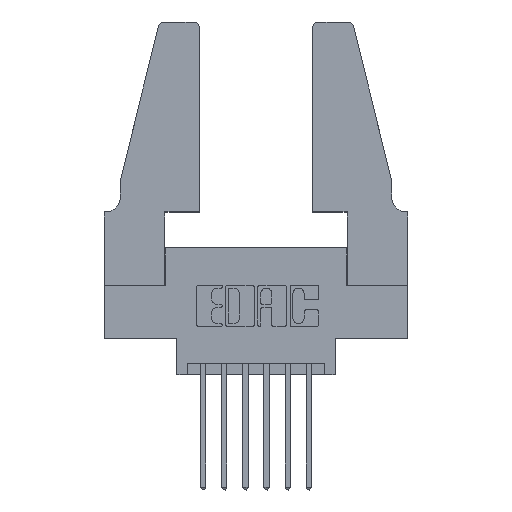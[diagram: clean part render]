
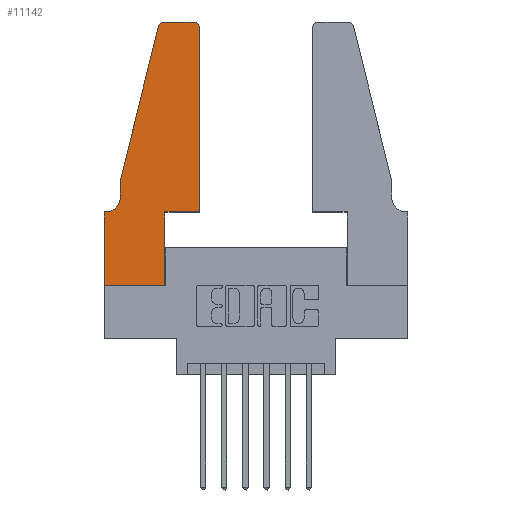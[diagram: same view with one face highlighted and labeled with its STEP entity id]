
A CAD part, top view. The second image highlights one B-rep face of the part: STEP entity #11142.
In plain terms, the highlighted planar face has unit normal (0, 0, 1).
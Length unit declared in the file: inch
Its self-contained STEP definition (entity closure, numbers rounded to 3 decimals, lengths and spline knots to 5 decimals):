
#231 = EDGE_CURVE ( 'NONE', #10431, #8152, #8017, .T. ) ;
#592 = VECTOR ( 'NONE', #11217, 39.37008 ) ;
#640 = DIRECTION ( 'NONE',  ( 0., 0., 1. ) ) ;
#743 = EDGE_CURVE ( 'NONE', #6571, #9268, #5655, .T. ) ;
#839 = CARTESIAN_POINT ( 'NONE',  ( 0.284, 1.22, 0.37 ) ) ;
#926 = EDGE_CURVE ( 'NONE', #6326, #11310, #8406, .T. ) ;
#970 = CARTESIAN_POINT ( 'NONE',  ( 0.0055, 0.42, 0.37 ) ) ;
#1036 = ORIENTED_EDGE ( 'NONE', *, *, #231, .T. ) ;
#1042 = VECTOR ( 'NONE', #9779, 39.37008 ) ;
#1610 = VERTEX_POINT ( 'NONE', #11147 ) ;
#1614 = FACE_OUTER_BOUND ( 'NONE', #6692, .T. ) ;
#1713 = DIRECTION ( 'NONE',  ( 0., 0., 1. ) ) ;
#1777 = DIRECTION ( 'NONE',  ( 1., 0., 0. ) ) ;
#1792 = VERTEX_POINT ( 'NONE', #5857 ) ;
#1813 = VERTEX_POINT ( 'NONE', #5241 ) ;
#1886 = DIRECTION ( 'NONE',  ( -0.239, -0.971, 0. ) ) ;
#1920 = DIRECTION ( 'NONE',  ( -1., 0., 0. ) ) ;
#1927 = CARTESIAN_POINT ( 'NONE',  ( 0.4505, 0.35, 0.37 ) ) ;
#1946 = EDGE_CURVE ( 'NONE', #9268, #1813, #5762, .T. ) ;
#2195 = VERTEX_POINT ( 'NONE', #5952 ) ;
#2462 = VECTOR ( 'NONE', #10970, 39.37008 ) ;
#2817 = EDGE_CURVE ( 'NONE', #7672, #1792, #4414, .T. ) ;
#2962 = ORIENTED_EDGE ( 'NONE', *, *, #7625, .T. ) ;
#3680 = VECTOR ( 'NONE', #4369, 39.37008 ) ;
#3730 = EDGE_CURVE ( 'NONE', #1792, #2195, #11265, .T. ) ;
#3849 = ORIENTED_EDGE ( 'NONE', *, *, #6217, .T. ) ;
#4110 = VECTOR ( 'NONE', #5999, 39.37008 ) ;
#4369 = DIRECTION ( 'NONE',  ( 0., -1., 0. ) ) ;
#4414 = LINE ( 'NONE', #6388, #4110 ) ;
#4507 = EDGE_CURVE ( 'NONE', #1610, #10431, #7741, .T. ) ;
#4512 = CARTESIAN_POINT ( 'NONE',  ( 0.0755, 0.5, 0.37 ) ) ;
#4696 = VERTEX_POINT ( 'NONE', #9492 ) ;
#4746 = ORIENTED_EDGE ( 'NONE', *, *, #2817, .T. ) ;
#5241 = CARTESIAN_POINT ( 'NONE',  ( 0., 0., 0.37 ) ) ;
#5282 = CARTESIAN_POINT ( 'NONE',  ( 0.0755, 0.5, 0.37 ) ) ;
#5295 = CARTESIAN_POINT ( 'NONE',  ( 0., 0.35, 0.37 ) ) ;
#5655 = LINE ( 'NONE', #8463, #592 ) ;
#5685 = AXIS2_PLACEMENT_3D ( 'NONE', #7307, #1713, #8178 ) ;
#5762 = LINE ( 'NONE', #6848, #10183 ) ;
#5857 = CARTESIAN_POINT ( 'NONE',  ( 0.4505, 1.22, 0.37 ) ) ;
#5952 = CARTESIAN_POINT ( 'NONE',  ( 0.4205, 1.25, 0.37 ) ) ;
#5999 = DIRECTION ( 'NONE',  ( 0., 1., 0. ) ) ;
#6182 = LINE ( 'NONE', #5282, #3680 ) ;
#6217 = EDGE_CURVE ( 'NONE', #8152, #4696, #6182, .T. ) ;
#6241 = AXIS2_PLACEMENT_3D ( 'NONE', #839, #7368, #1777 ) ;
#6295 = CARTESIAN_POINT ( 'NONE',  ( 0.4205, 1.22, 0.37 ) ) ;
#6326 = VERTEX_POINT ( 'NONE', #6355 ) ;
#6337 = ORIENTED_EDGE ( 'NONE', *, *, #11269, .T. ) ;
#6355 = CARTESIAN_POINT ( 'NONE',  ( 0.2865, 0., 0.37 ) ) ;
#6388 = CARTESIAN_POINT ( 'NONE',  ( 0.4505, 0.35, 0.37 ) ) ;
#6549 = VECTOR ( 'NONE', #6674, 39.37008 ) ;
#6561 = CARTESIAN_POINT ( 'NONE',  ( 0.2605, 1.25, 0.37 ) ) ;
#6571 = VERTEX_POINT ( 'NONE', #11098 ) ;
#6674 = DIRECTION ( 'NONE',  ( 1., 0., 0. ) ) ;
#6692 = EDGE_LOOP ( 'NONE', ( #2962, #10195, #1036, #3849, #6337, #11044, #8953, #11326, #9220, #11595, #4746, #7190 ) ) ;
#6774 = VECTOR ( 'NONE', #7971, 39.37008 ) ;
#6848 = CARTESIAN_POINT ( 'NONE',  ( 0., 0., 0.37 ) ) ;
#7104 = CARTESIAN_POINT ( 'NONE',  ( 0.4505, 0.35, 0.37 ) ) ;
#7190 = ORIENTED_EDGE ( 'NONE', *, *, #3730, .T. ) ;
#7198 = DIRECTION ( 'NONE',  ( 1., 0., 0. ) ) ;
#7307 = CARTESIAN_POINT ( 'NONE',  ( 0., 0.35, 0.37 ) ) ;
#7368 = DIRECTION ( 'NONE',  ( 0., 0., 1. ) ) ;
#7391 = LINE ( 'NONE', #6561, #2462 ) ;
#7485 = AXIS2_PLACEMENT_3D ( 'NONE', #6295, #640, #7198 ) ;
#7489 = DIRECTION ( 'NONE',  ( 0., 0., -1. ) ) ;
#7569 = CIRCLE ( 'NONE', #11024, 0.07 ) ;
#7625 = EDGE_CURVE ( 'NONE', #2195, #1610, #7391, .T. ) ;
#7672 = VERTEX_POINT ( 'NONE', #1927 ) ;
#7702 = EDGE_CURVE ( 'NONE', #1813, #6326, #9426, .T. ) ;
#7741 = CIRCLE ( 'NONE', #6241, 0.03 ) ;
#7971 = DIRECTION ( 'NONE',  ( 1., 0., 0. ) ) ;
#8017 = LINE ( 'NONE', #4512, #10084 ) ;
#8152 = VERTEX_POINT ( 'NONE', #11727 ) ;
#8178 = DIRECTION ( 'NONE',  ( 1., 0., 0. ) ) ;
#8406 = LINE ( 'NONE', #10836, #1042 ) ;
#8463 = CARTESIAN_POINT ( 'NONE',  ( 0.0755, 0.35, 0.37 ) ) ;
#8953 = ORIENTED_EDGE ( 'NONE', *, *, #1946, .T. ) ;
#9108 = LINE ( 'NONE', #7104, #6774 ) ;
#9220 = ORIENTED_EDGE ( 'NONE', *, *, #926, .T. ) ;
#9268 = VERTEX_POINT ( 'NONE', #5295 ) ;
#9426 = LINE ( 'NONE', #10181, #6549 ) ;
#9492 = CARTESIAN_POINT ( 'NONE',  ( 0.0755, 0.42, 0.37 ) ) ;
#9779 = DIRECTION ( 'NONE',  ( 0., 1., 0. ) ) ;
#9799 = EDGE_CURVE ( 'NONE', #11310, #7672, #9108, .T. ) ;
#10084 = VECTOR ( 'NONE', #1886, 39.37008 ) ;
#10178 = CARTESIAN_POINT ( 'NONE',  ( 0.2865, 0.35, 0.37 ) ) ;
#10181 = CARTESIAN_POINT ( 'NONE',  ( 0., 0., 0.37 ) ) ;
#10183 = VECTOR ( 'NONE', #11556, 39.37008 ) ;
#10195 = ORIENTED_EDGE ( 'NONE', *, *, #4507, .T. ) ;
#10431 = VERTEX_POINT ( 'NONE', #10592 ) ;
#10592 = CARTESIAN_POINT ( 'NONE',  ( 0.25487, 1.22718, 0.37 ) ) ;
#10811 = PLANE ( 'NONE',  #5685 ) ;
#10836 = CARTESIAN_POINT ( 'NONE',  ( 0.2865, 0.35, 0.37 ) ) ;
#10970 = DIRECTION ( 'NONE',  ( -1., 0., 0. ) ) ;
#11024 = AXIS2_PLACEMENT_3D ( 'NONE', #970, #7489, #1920 ) ;
#11044 = ORIENTED_EDGE ( 'NONE', *, *, #743, .T. ) ;
#11098 = CARTESIAN_POINT ( 'NONE',  ( 0.0055, 0.35, 0.37 ) ) ;
#11142 = ADVANCED_FACE ( 'NONE', ( #1614 ), #10811, .T. ) ;
#11147 = CARTESIAN_POINT ( 'NONE',  ( 0.284, 1.25, 0.37 ) ) ;
#11217 = DIRECTION ( 'NONE',  ( -1., 0., 0. ) ) ;
#11265 = CIRCLE ( 'NONE', #7485, 0.03 ) ;
#11269 = EDGE_CURVE ( 'NONE', #4696, #6571, #7569, .T. ) ;
#11310 = VERTEX_POINT ( 'NONE', #10178 ) ;
#11326 = ORIENTED_EDGE ( 'NONE', *, *, #7702, .T. ) ;
#11556 = DIRECTION ( 'NONE',  ( 0., -1., 0. ) ) ;
#11595 = ORIENTED_EDGE ( 'NONE', *, *, #9799, .T. ) ;
#11727 = CARTESIAN_POINT ( 'NONE',  ( 0.0755, 0.5, 0.37 ) ) ;
